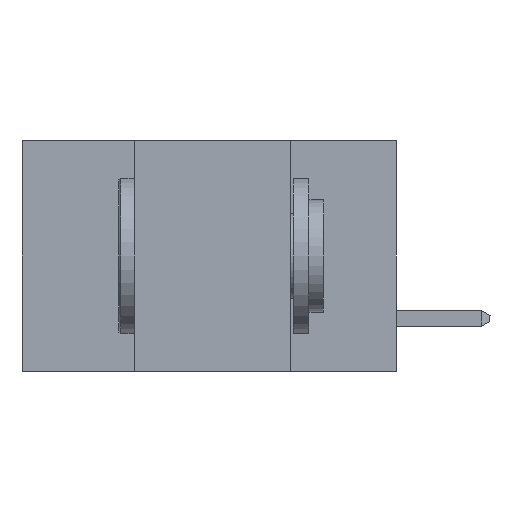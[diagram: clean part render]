
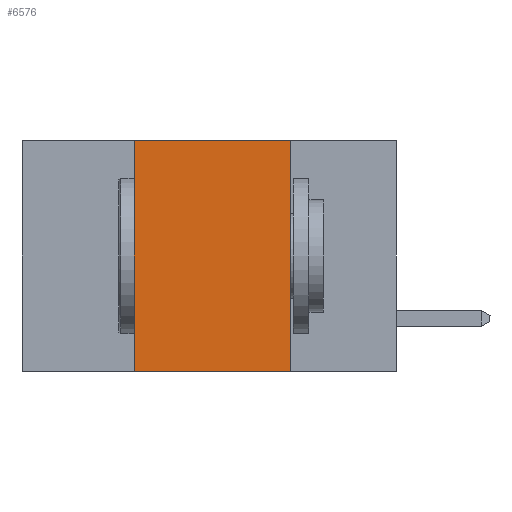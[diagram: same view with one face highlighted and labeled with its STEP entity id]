
A CAD part, left-side view. The second image highlights one B-rep face of the part: STEP entity #6576.
In plain terms, the highlighted planar face has unit normal (-1, 0, 0).
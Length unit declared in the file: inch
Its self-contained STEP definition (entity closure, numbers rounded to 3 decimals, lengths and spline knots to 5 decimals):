
#535 = DIRECTION ( 'NONE',  ( 0., 0., -1. ) ) ;
#786 = ORIENTED_EDGE ( 'NONE', *, *, #19444, .F. ) ;
#814 = VERTEX_POINT ( 'NONE', #2439 ) ;
#838 = DIRECTION ( 'NONE',  ( 0., 0., 1. ) ) ;
#2061 = ORIENTED_EDGE ( 'NONE', *, *, #12153, .T. ) ;
#2111 = CARTESIAN_POINT ( 'NONE',  ( 0., 0.6, 0. ) ) ;
#2269 = CARTESIAN_POINT ( 'NONE',  ( 0., 0.17, 0. ) ) ;
#2370 = CARTESIAN_POINT ( 'NONE',  ( 0., 0.6, -0.37 ) ) ;
#2439 = CARTESIAN_POINT ( 'NONE',  ( 0., 0.17, -0.37 ) ) ;
#3697 = DIRECTION ( 'NONE',  ( 0., -1., 0. ) ) ;
#3702 = CARTESIAN_POINT ( 'NONE',  ( 0., 0.6, 0. ) ) ;
#4018 = VERTEX_POINT ( 'NONE', #18142 ) ;
#6049 = FACE_OUTER_BOUND ( 'NONE', #10821, .T. ) ;
#6576 = ADVANCED_FACE ( 'NONE', ( #6049 ), #20171, .F. ) ;
#7024 = CARTESIAN_POINT ( 'NONE',  ( 0., 0.17, -0.37 ) ) ;
#7847 = VERTEX_POINT ( 'NONE', #8573 ) ;
#8238 = VECTOR ( 'NONE', #838, 39.37008 ) ;
#8573 = CARTESIAN_POINT ( 'NONE',  ( 0., 0.42, -0.37 ) ) ;
#8790 = LINE ( 'NONE', #2370, #20754 ) ;
#10117 = ORIENTED_EDGE ( 'NONE', *, *, #17177, .F. ) ;
#10379 = DIRECTION ( 'NONE',  ( 1., 0., 0. ) ) ;
#10808 = LINE ( 'NONE', #2111, #19060 ) ;
#10821 = EDGE_LOOP ( 'NONE', ( #10117, #11053, #786, #2061 ) ) ;
#11053 = ORIENTED_EDGE ( 'NONE', *, *, #12015, .F. ) ;
#11658 = LINE ( 'NONE', #7024, #15053 ) ;
#12015 = EDGE_CURVE ( 'NONE', #4018, #17264, #10808, .T. ) ;
#12153 = EDGE_CURVE ( 'NONE', #7847, #814, #8790, .T. ) ;
#12592 = LINE ( 'NONE', #13930, #8238 ) ;
#13930 = CARTESIAN_POINT ( 'NONE',  ( 0., 0.42, -0.37 ) ) ;
#15053 = VECTOR ( 'NONE', #15305, 39.37008 ) ;
#15305 = DIRECTION ( 'NONE',  ( 0., 0., -1. ) ) ;
#17177 = EDGE_CURVE ( 'NONE', #17264, #814, #11658, .T. ) ;
#17264 = VERTEX_POINT ( 'NONE', #2269 ) ;
#18142 = CARTESIAN_POINT ( 'NONE',  ( 0., 0.42, 0. ) ) ;
#19060 = VECTOR ( 'NONE', #3697, 39.37008 ) ;
#19444 = EDGE_CURVE ( 'NONE', #7847, #4018, #12592, .T. ) ;
#19472 = AXIS2_PLACEMENT_3D ( 'NONE', #3702, #10379, #535 ) ;
#20171 = PLANE ( 'NONE',  #19472 ) ;
#20369 = DIRECTION ( 'NONE',  ( 0., -1., 0. ) ) ;
#20754 = VECTOR ( 'NONE', #20369, 39.37008 ) ;
